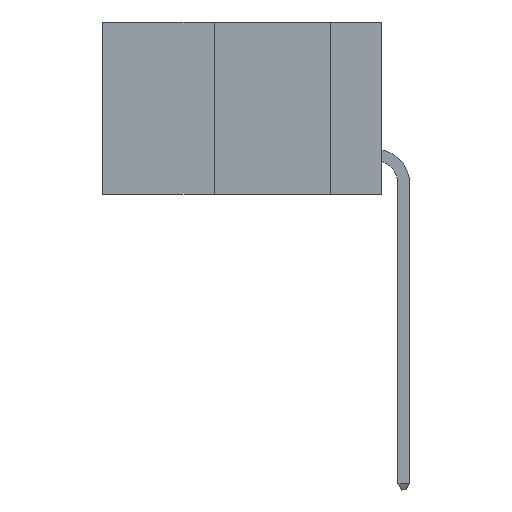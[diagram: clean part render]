
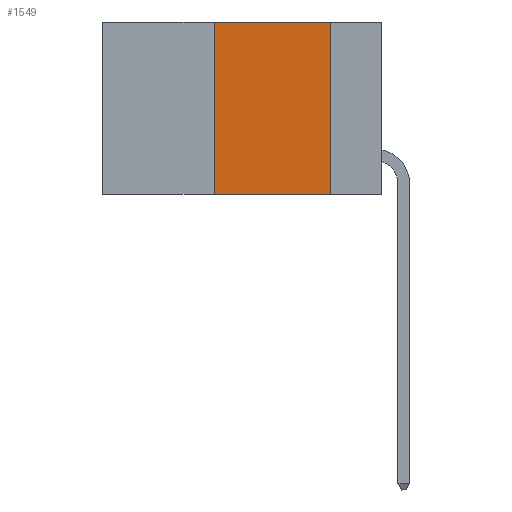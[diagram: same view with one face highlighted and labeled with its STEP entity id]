
A CAD part, left-side view. The second image highlights one B-rep face of the part: STEP entity #1549.
In plain terms, the highlighted planar face has unit normal (-1, 0, 0).
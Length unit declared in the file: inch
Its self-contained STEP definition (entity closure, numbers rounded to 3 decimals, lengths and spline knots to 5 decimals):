
#1549 = ADVANCED_FACE ( 'NONE', ( #21167 ), #14581, .F. ) ;
#2014 = ORIENTED_EDGE ( 'NONE', *, *, #2979, .F. ) ;
#2134 = CARTESIAN_POINT ( 'NONE',  ( 0., 0.6, -0.37 ) ) ;
#2182 = DIRECTION ( 'NONE',  ( 0., 0., -1. ) ) ;
#2204 = DIRECTION ( 'NONE',  ( 0., -1., 0. ) ) ;
#2758 = ORIENTED_EDGE ( 'NONE', *, *, #15985, .F. ) ;
#2979 = EDGE_CURVE ( 'NONE', #12156, #20753, #19270, .T. ) ;
#3017 = DIRECTION ( 'NONE',  ( 0., 0., -1. ) ) ;
#3241 = VECTOR ( 'NONE', #2182, 39.37008 ) ;
#4380 = EDGE_CURVE ( 'NONE', #20916, #13354, #19466, .T. ) ;
#6366 = CARTESIAN_POINT ( 'NONE',  ( 0., 0.11, -0.37 ) ) ;
#6410 = CARTESIAN_POINT ( 'NONE',  ( 0., 0.6, 0. ) ) ;
#9142 = LINE ( 'NONE', #12214, #10925 ) ;
#9735 = CARTESIAN_POINT ( 'NONE',  ( 0., 0.6, 0. ) ) ;
#10826 = ORIENTED_EDGE ( 'NONE', *, *, #4380, .T. ) ;
#10925 = VECTOR ( 'NONE', #13964, 39.37008 ) ;
#12156 = VERTEX_POINT ( 'NONE', #15119 ) ;
#12214 = CARTESIAN_POINT ( 'NONE',  ( 0., 0.36, 0. ) ) ;
#12547 = EDGE_LOOP ( 'NONE', ( #2758, #2014, #18214, #10826 ) ) ;
#13354 = VERTEX_POINT ( 'NONE', #6366 ) ;
#13964 = DIRECTION ( 'NONE',  ( 0., 0., 1. ) ) ;
#14581 = PLANE ( 'NONE',  #17278 ) ;
#15119 = CARTESIAN_POINT ( 'NONE',  ( 0., 0.36, 0. ) ) ;
#15289 = VECTOR ( 'NONE', #16385, 39.37008 ) ;
#15364 = LINE ( 'NONE', #17950, #3241 ) ;
#15474 = CARTESIAN_POINT ( 'NONE',  ( 0., 0.36, -0.37 ) ) ;
#15985 = EDGE_CURVE ( 'NONE', #20753, #13354, #15364, .T. ) ;
#16241 = CARTESIAN_POINT ( 'NONE',  ( 0., 0.11, 0. ) ) ;
#16374 = DIRECTION ( 'NONE',  ( 1., 0., 0. ) ) ;
#16385 = DIRECTION ( 'NONE',  ( 0., -1., 0. ) ) ;
#17278 = AXIS2_PLACEMENT_3D ( 'NONE', #6410, #16374, #3017 ) ;
#17950 = CARTESIAN_POINT ( 'NONE',  ( 0., 0.11, 0. ) ) ;
#18214 = ORIENTED_EDGE ( 'NONE', *, *, #18825, .F. ) ;
#18825 = EDGE_CURVE ( 'NONE', #20916, #12156, #9142, .T. ) ;
#19270 = LINE ( 'NONE', #9735, #15289 ) ;
#19466 = LINE ( 'NONE', #2134, #20527 ) ;
#20527 = VECTOR ( 'NONE', #2204, 39.37008 ) ;
#20753 = VERTEX_POINT ( 'NONE', #16241 ) ;
#20916 = VERTEX_POINT ( 'NONE', #15474 ) ;
#21167 = FACE_OUTER_BOUND ( 'NONE', #12547, .T. ) ;
